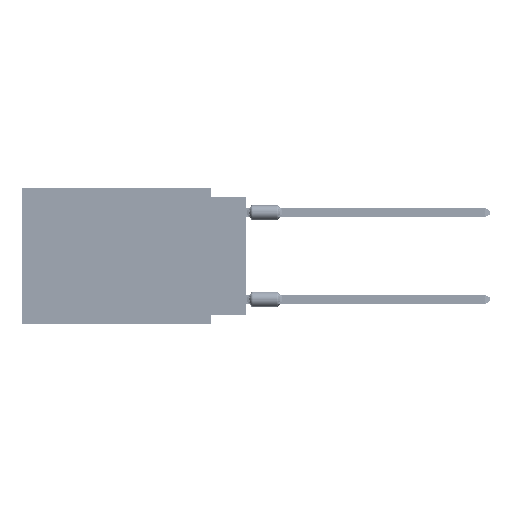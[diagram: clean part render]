
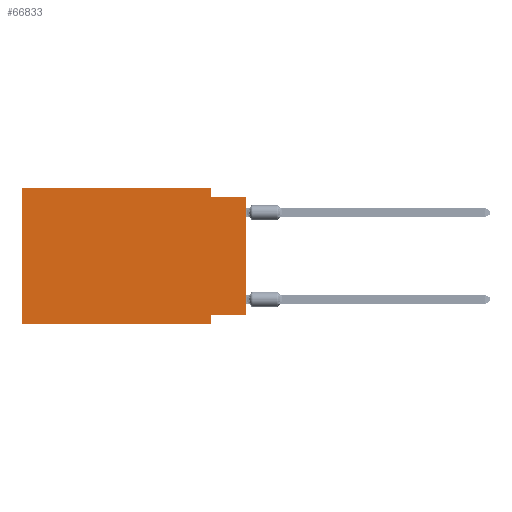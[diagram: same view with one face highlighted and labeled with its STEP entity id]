
A CAD part, left-side view. The second image highlights one B-rep face of the part: STEP entity #66833.
In plain terms, the highlighted planar face has unit normal (-1, 0, 0).
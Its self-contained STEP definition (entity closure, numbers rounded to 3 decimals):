
#724 = CARTESIAN_POINT ( 'NONE',  ( 0., 0., 0. ) ) ;
#1049 = VERTEX_POINT ( 'NONE', #68332 ) ;
#1620 = VECTOR ( 'NONE', #43543, 1000. ) ;
#2023 = FACE_OUTER_BOUND ( 'NONE', #25273, .T. ) ;
#2360 = LINE ( 'NONE', #14439, #19039 ) ;
#2390 = DIRECTION ( 'NONE',  ( 1., 0., 0. ) ) ;
#2682 = ORIENTED_EDGE ( 'NONE', *, *, #56133, .T. ) ;
#2802 = ORIENTED_EDGE ( 'NONE', *, *, #21589, .F. ) ;
#6165 = VERTEX_POINT ( 'NONE', #37397 ) ;
#6281 = LINE ( 'NONE', #40635, #53616 ) ;
#7300 = CARTESIAN_POINT ( 'NONE',  ( 0., 0., -0.635 ) ) ;
#7508 = DIRECTION ( 'NONE',  ( 0., 0., 1. ) ) ;
#8238 = LINE ( 'NONE', #31252, #68978 ) ;
#8831 = CARTESIAN_POINT ( 'NONE',  ( 0., 2.54, 0. ) ) ;
#13124 = VERTEX_POINT ( 'NONE', #34824 ) ;
#13389 = LINE ( 'NONE', #8831, #1620 ) ;
#13760 = LINE ( 'NONE', #25432, #31799 ) ;
#14439 = CARTESIAN_POINT ( 'NONE',  ( 0., 16.383, -9.906 ) ) ;
#16269 = VECTOR ( 'NONE', #39408, 1000. ) ;
#16770 = LINE ( 'NONE', #45819, #16269 ) ;
#18681 = VERTEX_POINT ( 'NONE', #52075 ) ;
#19039 = VECTOR ( 'NONE', #60485, 1000. ) ;
#19745 = EDGE_CURVE ( 'NONE', #65854, #6165, #13760, .T. ) ;
#19757 = PLANE ( 'NONE',  #35706 ) ;
#19782 = DIRECTION ( 'NONE',  ( 0., 1., 0. ) ) ;
#19806 = EDGE_CURVE ( 'NONE', #69653, #60244, #13389, .T. ) ;
#20210 = CARTESIAN_POINT ( 'NONE',  ( 0., 2.54, 0. ) ) ;
#21589 = EDGE_CURVE ( 'NONE', #6165, #13124, #16770, .T. ) ;
#21720 = VERTEX_POINT ( 'NONE', #7300 ) ;
#25273 = EDGE_LOOP ( 'NONE', ( #29517, #65093, #56088, #72836, #27530, #2682, #2802, #53588 ) ) ;
#25432 = CARTESIAN_POINT ( 'NONE',  ( 0., 0., -9.271 ) ) ;
#27530 = ORIENTED_EDGE ( 'NONE', *, *, #68764, .F. ) ;
#29517 = ORIENTED_EDGE ( 'NONE', *, *, #30100, .T. ) ;
#29789 = LINE ( 'NONE', #724, #58567 ) ;
#30100 = EDGE_CURVE ( 'NONE', #65854, #21720, #29789, .T. ) ;
#31252 = CARTESIAN_POINT ( 'NONE',  ( 0., 0., -0.635 ) ) ;
#31799 = VECTOR ( 'NONE', #19782, 1000. ) ;
#32189 = CARTESIAN_POINT ( 'NONE',  ( 0., 0., -9.271 ) ) ;
#34824 = CARTESIAN_POINT ( 'NONE',  ( 0., 2.54, -9.906 ) ) ;
#35254 = CARTESIAN_POINT ( 'NONE',  ( 0., 16.383, 0. ) ) ;
#35706 = AXIS2_PLACEMENT_3D ( 'NONE', #54473, #2390, #70357 ) ;
#37397 = CARTESIAN_POINT ( 'NONE',  ( 0., 2.54, -9.271 ) ) ;
#39408 = DIRECTION ( 'NONE',  ( 0., 0., -1. ) ) ;
#40635 = CARTESIAN_POINT ( 'NONE',  ( 0., 16.383, 0. ) ) ;
#41086 = CARTESIAN_POINT ( 'NONE',  ( 0., 2.54, -0.635 ) ) ;
#43543 = DIRECTION ( 'NONE',  ( 0., 0., -1. ) ) ;
#44851 = EDGE_CURVE ( 'NONE', #1049, #69653, #6281, .T. ) ;
#45819 = CARTESIAN_POINT ( 'NONE',  ( 0., 2.54, -9.906 ) ) ;
#51586 = DIRECTION ( 'NONE',  ( 0., -1., 0. ) ) ;
#52075 = CARTESIAN_POINT ( 'NONE',  ( 0., 16.383, -9.906 ) ) ;
#53588 = ORIENTED_EDGE ( 'NONE', *, *, #19745, .F. ) ;
#53616 = VECTOR ( 'NONE', #51586, 1000. ) ;
#54272 = EDGE_CURVE ( 'NONE', #60244, #21720, #8238, .T. ) ;
#54277 = DIRECTION ( 'NONE',  ( 0., -1., 0. ) ) ;
#54473 = CARTESIAN_POINT ( 'NONE',  ( 0., 16.383, 0. ) ) ;
#56088 = ORIENTED_EDGE ( 'NONE', *, *, #19806, .F. ) ;
#56133 = EDGE_CURVE ( 'NONE', #18681, #13124, #2360, .T. ) ;
#57521 = LINE ( 'NONE', #35254, #65868 ) ;
#58567 = VECTOR ( 'NONE', #7508, 1000. ) ;
#60244 = VERTEX_POINT ( 'NONE', #41086 ) ;
#60485 = DIRECTION ( 'NONE',  ( 0., -1., 0. ) ) ;
#65093 = ORIENTED_EDGE ( 'NONE', *, *, #54272, .F. ) ;
#65854 = VERTEX_POINT ( 'NONE', #32189 ) ;
#65868 = VECTOR ( 'NONE', #74132, 1000. ) ;
#66833 = ADVANCED_FACE ( 'NONE', ( #2023 ), #19757, .F. ) ;
#68332 = CARTESIAN_POINT ( 'NONE',  ( 0., 16.383, 0. ) ) ;
#68764 = EDGE_CURVE ( 'NONE', #18681, #1049, #57521, .T. ) ;
#68978 = VECTOR ( 'NONE', #54277, 1000. ) ;
#69653 = VERTEX_POINT ( 'NONE', #20210 ) ;
#70357 = DIRECTION ( 'NONE',  ( 0., 0., -1. ) ) ;
#72836 = ORIENTED_EDGE ( 'NONE', *, *, #44851, .F. ) ;
#74132 = DIRECTION ( 'NONE',  ( 0., 0., 1. ) ) ;
